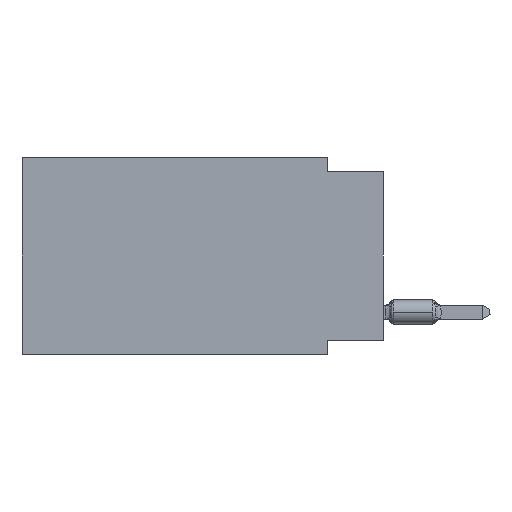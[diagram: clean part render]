
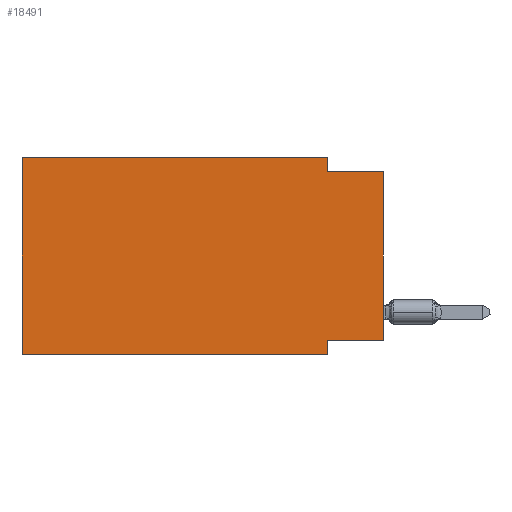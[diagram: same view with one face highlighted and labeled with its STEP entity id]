
A CAD part, left-side view. The second image highlights one B-rep face of the part: STEP entity #18491.
In plain terms, the highlighted planar face has unit normal (-1, 0, 0).
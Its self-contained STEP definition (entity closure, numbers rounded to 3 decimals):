
#1963 = CARTESIAN_POINT ( 'NONE',  ( 0., 16.383, 0. ) ) ;
#2901 = LINE ( 'NONE', #31497, #66656 ) ;
#3123 = DIRECTION ( 'NONE',  ( 0., 0., 1. ) ) ;
#4237 = CARTESIAN_POINT ( 'NONE',  ( 0., 16.383, 0. ) ) ;
#4679 = CARTESIAN_POINT ( 'NONE',  ( 0., 0., -8.255 ) ) ;
#5050 = ORIENTED_EDGE ( 'NONE', *, *, #25440, .F. ) ;
#7827 = LINE ( 'NONE', #66548, #26784 ) ;
#8198 = EDGE_CURVE ( 'NONE', #50846, #60877, #52324, .T. ) ;
#8843 = LINE ( 'NONE', #72150, #18218 ) ;
#9650 = EDGE_CURVE ( 'NONE', #50846, #37480, #8843, .T. ) ;
#10059 = EDGE_LOOP ( 'NONE', ( #59168, #60513, #37157, #31620, #18293, #65096, #5050, #14836 ) ) ;
#12625 = FACE_OUTER_BOUND ( 'NONE', #10059, .T. ) ;
#14836 = ORIENTED_EDGE ( 'NONE', *, *, #8198, .F. ) ;
#15245 = CARTESIAN_POINT ( 'NONE',  ( 0., 2.54, -8.89 ) ) ;
#15409 = DIRECTION ( 'NONE',  ( 0., 0., 1. ) ) ;
#17243 = DIRECTION ( 'NONE',  ( 0., 1., 0. ) ) ;
#18218 = VECTOR ( 'NONE', #3123, 1000. ) ;
#18225 = VECTOR ( 'NONE', #17243, 1000. ) ;
#18293 = ORIENTED_EDGE ( 'NONE', *, *, #55828, .F. ) ;
#18351 = CARTESIAN_POINT ( 'NONE',  ( 0., 0., -0.635 ) ) ;
#18491 = ADVANCED_FACE ( 'NONE', ( #12625 ), #48483, .F. ) ;
#19178 = CARTESIAN_POINT ( 'NONE',  ( 0., 0., -8.255 ) ) ;
#21861 = LINE ( 'NONE', #39030, #50238 ) ;
#24452 = VECTOR ( 'NONE', #68674, 1000. ) ;
#25214 = DIRECTION ( 'NONE',  ( 1., 0., 0. ) ) ;
#25440 = EDGE_CURVE ( 'NONE', #60877, #52613, #21861, .T. ) ;
#26784 = VECTOR ( 'NONE', #15409, 1000. ) ;
#27553 = CARTESIAN_POINT ( 'NONE',  ( 0., 16.383, -8.89 ) ) ;
#28812 = VERTEX_POINT ( 'NONE', #45473 ) ;
#29811 = VECTOR ( 'NONE', #57591, 1000. ) ;
#30612 = EDGE_CURVE ( 'NONE', #40154, #48813, #45402, .T. ) ;
#31497 = CARTESIAN_POINT ( 'NONE',  ( 0., 0., -0.635 ) ) ;
#31620 = ORIENTED_EDGE ( 'NONE', *, *, #68354, .F. ) ;
#34783 = LINE ( 'NONE', #27553, #69545 ) ;
#37157 = ORIENTED_EDGE ( 'NONE', *, *, #30612, .F. ) ;
#37480 = VERTEX_POINT ( 'NONE', #18351 ) ;
#39030 = CARTESIAN_POINT ( 'NONE',  ( 0., 2.54, -8.89 ) ) ;
#40154 = VERTEX_POINT ( 'NONE', #41320 ) ;
#41320 = CARTESIAN_POINT ( 'NONE',  ( 0., 2.54, 0. ) ) ;
#42038 = CARTESIAN_POINT ( 'NONE',  ( 0., 16.383, 0. ) ) ;
#44296 = LINE ( 'NONE', #4237, #24452 ) ;
#45402 = LINE ( 'NONE', #58339, #29811 ) ;
#45473 = CARTESIAN_POINT ( 'NONE',  ( 0., 16.383, -8.89 ) ) ;
#48483 = PLANE ( 'NONE',  #68900 ) ;
#48813 = VERTEX_POINT ( 'NONE', #65133 ) ;
#50238 = VECTOR ( 'NONE', #62280, 1000. ) ;
#50846 = VERTEX_POINT ( 'NONE', #19178 ) ;
#52324 = LINE ( 'NONE', #4679, #18225 ) ;
#52613 = VERTEX_POINT ( 'NONE', #15245 ) ;
#53449 = EDGE_CURVE ( 'NONE', #48813, #37480, #2901, .T. ) ;
#55828 = EDGE_CURVE ( 'NONE', #28812, #63652, #7827, .T. ) ;
#57591 = DIRECTION ( 'NONE',  ( 0., 0., -1. ) ) ;
#58339 = CARTESIAN_POINT ( 'NONE',  ( 0., 2.54, 0. ) ) ;
#59168 = ORIENTED_EDGE ( 'NONE', *, *, #9650, .T. ) ;
#59411 = CARTESIAN_POINT ( 'NONE',  ( 0., 2.54, -8.255 ) ) ;
#60513 = ORIENTED_EDGE ( 'NONE', *, *, #53449, .F. ) ;
#60877 = VERTEX_POINT ( 'NONE', #59411 ) ;
#61220 = DIRECTION ( 'NONE',  ( 0., -1., 0. ) ) ;
#62280 = DIRECTION ( 'NONE',  ( 0., 0., -1. ) ) ;
#63652 = VERTEX_POINT ( 'NONE', #42038 ) ;
#64493 = DIRECTION ( 'NONE',  ( 0., 0., -1. ) ) ;
#65096 = ORIENTED_EDGE ( 'NONE', *, *, #72872, .T. ) ;
#65133 = CARTESIAN_POINT ( 'NONE',  ( 0., 2.54, -0.635 ) ) ;
#66548 = CARTESIAN_POINT ( 'NONE',  ( 0., 16.383, 0. ) ) ;
#66656 = VECTOR ( 'NONE', #61220, 1000. ) ;
#68354 = EDGE_CURVE ( 'NONE', #63652, #40154, #44296, .T. ) ;
#68674 = DIRECTION ( 'NONE',  ( 0., -1., 0. ) ) ;
#68900 = AXIS2_PLACEMENT_3D ( 'NONE', #1963, #25214, #64493 ) ;
#69545 = VECTOR ( 'NONE', #73711, 1000. ) ;
#72150 = CARTESIAN_POINT ( 'NONE',  ( 0., 0., 0. ) ) ;
#72872 = EDGE_CURVE ( 'NONE', #28812, #52613, #34783, .T. ) ;
#73711 = DIRECTION ( 'NONE',  ( 0., -1., 0. ) ) ;
